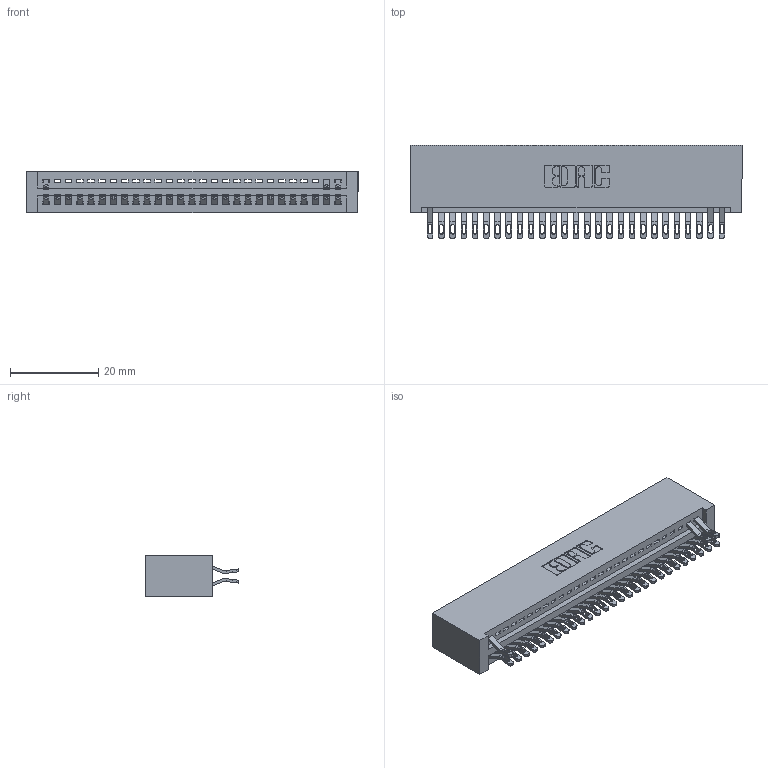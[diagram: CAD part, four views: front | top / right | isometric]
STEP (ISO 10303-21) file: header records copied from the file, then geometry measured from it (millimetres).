
FILE_DESCRIPTION (( 'STEP AP203' ), '1' );
FILE_NAME ('345-054-555-201.STEP', '2018-09-24T00:27:57', ( '' ), ( '' ), 'SwSTEP 2.0', 'SolidWorks 2016', '' );
FILE_SCHEMA (( 'CONFIG_CONTROL_DESIGN' ));
Length unit declared in the file: inch
Products named in the file (3): 345 Part_No Mounting Lugs; 345-292-001_555 Tail; 345-054-555-201
Assembly tree (31 placements, depth 2):
  345-054-555-201
    345 Part_No Mounting Lugs
    345-292-001_555 Tail  x30
Bounding box: 75.18 x 21.13 x 9.4 mm (x, y, z)
Volume: 7650.8 mm3; surface area: 10399.3 mm2
Topology: 31 solids, 31 shells, 1990 faces, 6275 edges, 4182 vertices
Faces by surface type: plane 1174, cylinder 816
Entity records: 22485 total; most frequent: CARTESIAN_POINT 3922, ORIENTED_EDGE 3850, DIRECTION 3413, EDGE_CURVE 1925, LINE 1673, VECTOR 1673, VERTEX_POINT 1282, AXIS2_PLACEMENT_3D 870
